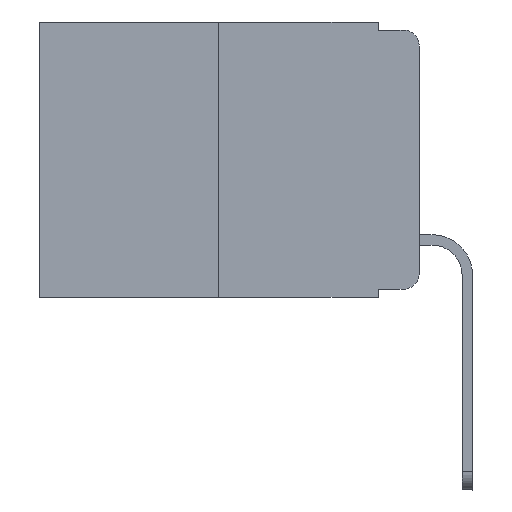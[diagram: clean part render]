
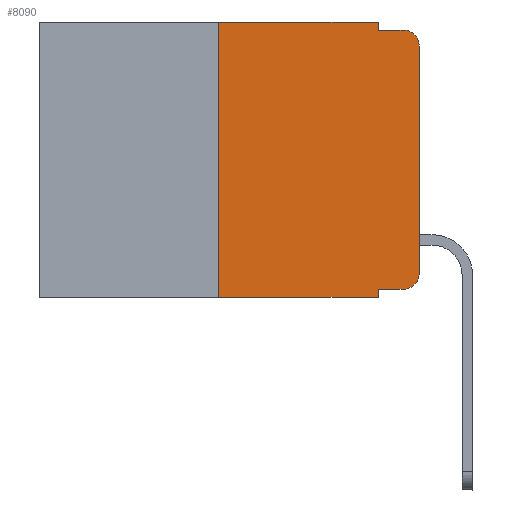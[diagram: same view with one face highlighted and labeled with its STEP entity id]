
A CAD part, left-side view. The second image highlights one B-rep face of the part: STEP entity #8090.
In plain terms, the highlighted planar face has unit normal (-1, 0, 0).
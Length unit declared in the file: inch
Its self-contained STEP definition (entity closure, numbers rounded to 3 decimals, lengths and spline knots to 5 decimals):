
#7 = ORIENTED_EDGE ( 'NONE', *, *, #11877, .T. ) ;
#326 = CARTESIAN_POINT ( 'NONE',  ( 0., 0.25, -0.343 ) ) ;
#397 = EDGE_LOOP ( 'NONE', ( #13971, #21179, #6225, #5650, #17092, #9394, #806, #9817, #7, #450 ) ) ;
#408 = EDGE_CURVE ( 'NONE', #6961, #16207, #10227, .T. ) ;
#450 = ORIENTED_EDGE ( 'NONE', *, *, #18612, .T. ) ;
#557 = CARTESIAN_POINT ( 'NONE',  ( 0., 0.051, -0.333 ) ) ;
#652 = DIRECTION ( 'NONE',  ( -1., 0., 0. ) ) ;
#692 = DIRECTION ( 'NONE',  ( -1., 0., 0. ) ) ;
#806 = ORIENTED_EDGE ( 'NONE', *, *, #18781, .T. ) ;
#1045 = FACE_OUTER_BOUND ( 'NONE', #397, .T. ) ;
#1455 = CARTESIAN_POINT ( 'NONE',  ( 0., 0.051, -0.333 ) ) ;
#1548 = LINE ( 'NONE', #14659, #12463 ) ;
#2698 = LINE ( 'NONE', #14297, #15957 ) ;
#2890 = DIRECTION ( 'NONE',  ( 0., 0., -1. ) ) ;
#3147 = VERTEX_POINT ( 'NONE', #4279 ) ;
#3620 = CARTESIAN_POINT ( 'NONE',  ( 0., 0., -0.03 ) ) ;
#4274 = CARTESIAN_POINT ( 'NONE',  ( 0., 0.473, -0.343 ) ) ;
#4279 = CARTESIAN_POINT ( 'NONE',  ( 0., 0.051, -0.343 ) ) ;
#4435 = VECTOR ( 'NONE', #10878, 39.37008 ) ;
#4895 = VERTEX_POINT ( 'NONE', #19135 ) ;
#5650 = ORIENTED_EDGE ( 'NONE', *, *, #10823, .F. ) ;
#5736 = CARTESIAN_POINT ( 'NONE',  ( 0., 0.02, -0.03 ) ) ;
#6106 = LINE ( 'NONE', #4274, #4435 ) ;
#6126 = DIRECTION ( 'NONE',  ( 1., 0., 0. ) ) ;
#6225 = ORIENTED_EDGE ( 'NONE', *, *, #15440, .F. ) ;
#6268 = CARTESIAN_POINT ( 'NONE',  ( 0., 0.02, -0.333 ) ) ;
#6336 = DIRECTION ( 'NONE',  ( 0., 0., 1. ) ) ;
#6956 = DIRECTION ( 'NONE',  ( 0., -1., 0. ) ) ;
#6961 = VERTEX_POINT ( 'NONE', #326 ) ;
#7077 = VERTEX_POINT ( 'NONE', #13770 ) ;
#7170 = VECTOR ( 'NONE', #21243, 39.37008 ) ;
#7253 = DIRECTION ( 'NONE',  ( 0., 0., -1. ) ) ;
#7291 = DIRECTION ( 'NONE',  ( 0., 0., 1. ) ) ;
#7300 = DIRECTION ( 'NONE',  ( 0., 0., -1. ) ) ;
#7564 = DIRECTION ( 'NONE',  ( 0., -1., 0. ) ) ;
#7644 = PLANE ( 'NONE',  #21371 ) ;
#8090 = ADVANCED_FACE ( 'NONE', ( #1045 ), #7644, .F. ) ;
#8170 = LINE ( 'NONE', #13062, #19732 ) ;
#8906 = AXIS2_PLACEMENT_3D ( 'NONE', #16829, #692, #7300 ) ;
#9394 = ORIENTED_EDGE ( 'NONE', *, *, #408, .F. ) ;
#9407 = VERTEX_POINT ( 'NONE', #13962 ) ;
#9523 = VERTEX_POINT ( 'NONE', #6268 ) ;
#9817 = ORIENTED_EDGE ( 'NONE', *, *, #13477, .F. ) ;
#9856 = LINE ( 'NONE', #14639, #17297 ) ;
#10227 = LINE ( 'NONE', #13918, #15532 ) ;
#10823 = EDGE_CURVE ( 'NONE', #7077, #11906, #14509, .T. ) ;
#10878 = DIRECTION ( 'NONE',  ( 0., -1., 0. ) ) ;
#11281 = DIRECTION ( 'NONE',  ( 0., -1., 0. ) ) ;
#11877 = EDGE_CURVE ( 'NONE', #13461, #9523, #16918, .T. ) ;
#11906 = VERTEX_POINT ( 'NONE', #12270 ) ;
#12270 = CARTESIAN_POINT ( 'NONE',  ( 0., 0.051, -0.01 ) ) ;
#12446 = EDGE_CURVE ( 'NONE', #20753, #4895, #15197, .T. ) ;
#12463 = VECTOR ( 'NONE', #21063, 39.37008 ) ;
#13011 = EDGE_CURVE ( 'NONE', #9407, #20753, #8170, .T. ) ;
#13062 = CARTESIAN_POINT ( 'NONE',  ( 0., 0., 0. ) ) ;
#13461 = VERTEX_POINT ( 'NONE', #1455 ) ;
#13477 = EDGE_CURVE ( 'NONE', #13461, #3147, #1548, .T. ) ;
#13770 = CARTESIAN_POINT ( 'NONE',  ( 0., 0.051, 0. ) ) ;
#13911 = CARTESIAN_POINT ( 'NONE',  ( 0., 0.25, 0. ) ) ;
#13918 = CARTESIAN_POINT ( 'NONE',  ( 0., 0.25, 0. ) ) ;
#13962 = CARTESIAN_POINT ( 'NONE',  ( 0., 0., -0.313 ) ) ;
#13971 = ORIENTED_EDGE ( 'NONE', *, *, #13011, .T. ) ;
#14297 = CARTESIAN_POINT ( 'NONE',  ( 0., 0.051, -0.01 ) ) ;
#14509 = LINE ( 'NONE', #16025, #7170 ) ;
#14639 = CARTESIAN_POINT ( 'NONE',  ( 0., 0.473, 0. ) ) ;
#14659 = CARTESIAN_POINT ( 'NONE',  ( 0., 0.051, 0. ) ) ;
#15146 = CIRCLE ( 'NONE', #8906, 0.02 ) ;
#15197 = CIRCLE ( 'NONE', #17247, 0.02 ) ;
#15235 = EDGE_CURVE ( 'NONE', #16207, #7077, #9856, .T. ) ;
#15440 = EDGE_CURVE ( 'NONE', #11906, #4895, #2698, .T. ) ;
#15532 = VECTOR ( 'NONE', #7291, 39.37008 ) ;
#15957 = VECTOR ( 'NONE', #7564, 39.37008 ) ;
#16025 = CARTESIAN_POINT ( 'NONE',  ( 0., 0.051, 0. ) ) ;
#16207 = VERTEX_POINT ( 'NONE', #13911 ) ;
#16829 = CARTESIAN_POINT ( 'NONE',  ( 0., 0.02, -0.313 ) ) ;
#16918 = LINE ( 'NONE', #557, #19695 ) ;
#17092 = ORIENTED_EDGE ( 'NONE', *, *, #15235, .F. ) ;
#17247 = AXIS2_PLACEMENT_3D ( 'NONE', #5736, #652, #7253 ) ;
#17297 = VECTOR ( 'NONE', #11281, 39.37008 ) ;
#18612 = EDGE_CURVE ( 'NONE', #9523, #9407, #15146, .T. ) ;
#18781 = EDGE_CURVE ( 'NONE', #6961, #3147, #6106, .T. ) ;
#19135 = CARTESIAN_POINT ( 'NONE',  ( 0., 0.02, -0.01 ) ) ;
#19695 = VECTOR ( 'NONE', #6956, 39.37008 ) ;
#19732 = VECTOR ( 'NONE', #6336, 39.37008 ) ;
#20753 = VERTEX_POINT ( 'NONE', #3620 ) ;
#20977 = CARTESIAN_POINT ( 'NONE',  ( 0., 0.473, 0. ) ) ;
#21063 = DIRECTION ( 'NONE',  ( 0., 0., -1. ) ) ;
#21179 = ORIENTED_EDGE ( 'NONE', *, *, #12446, .T. ) ;
#21243 = DIRECTION ( 'NONE',  ( 0., 0., -1. ) ) ;
#21371 = AXIS2_PLACEMENT_3D ( 'NONE', #20977, #6126, #2890 ) ;
